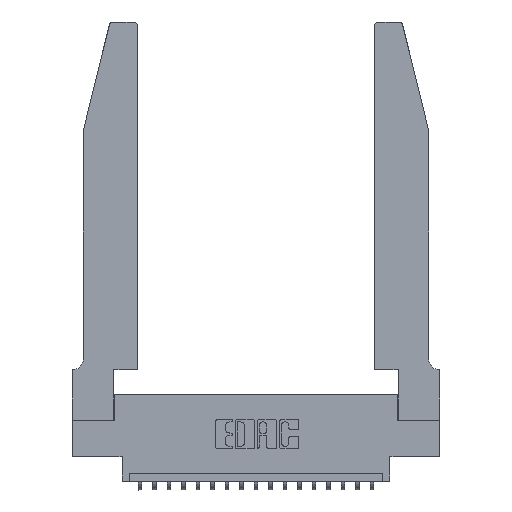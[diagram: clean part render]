
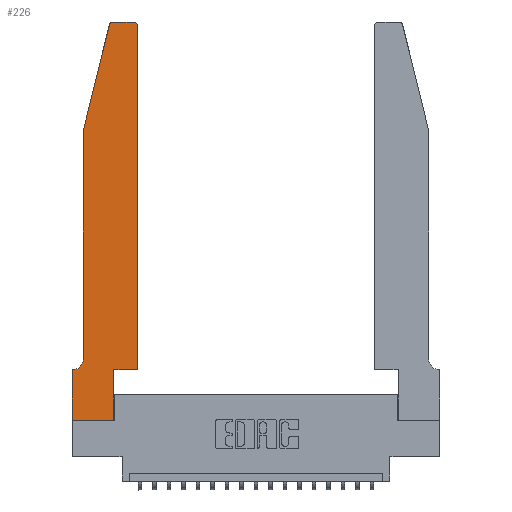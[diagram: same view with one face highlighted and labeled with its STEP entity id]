
A CAD part, top view. The second image highlights one B-rep face of the part: STEP entity #226.
In plain terms, the highlighted planar face has unit normal (0, 0, 1).
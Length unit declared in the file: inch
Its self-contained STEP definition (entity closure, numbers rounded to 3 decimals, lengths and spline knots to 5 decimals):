
#226 = ADVANCED_FACE ( 'NONE', ( #11697 ), #6208, .T. ) ;
#613 = CARTESIAN_POINT ( 'NONE',  ( 0.0055, 0.35, 0.37 ) ) ;
#615 = CARTESIAN_POINT ( 'NONE',  ( 0.4205, 2.75, 0.37 ) ) ;
#925 = DIRECTION ( 'NONE',  ( 0., 1., 0. ) ) ;
#1300 = CARTESIAN_POINT ( 'NONE',  ( 0.0755, 0.42, 0.37 ) ) ;
#1476 = AXIS2_PLACEMENT_3D ( 'NONE', #11097, #6129, #6274 ) ;
#2046 = ORIENTED_EDGE ( 'NONE', *, *, #7264, .T. ) ;
#2271 = EDGE_CURVE ( 'NONE', #5523, #13299, #11342, .T. ) ;
#2970 = CARTESIAN_POINT ( 'NONE',  ( 0.0755, 2., 0.37 ) ) ;
#3034 = EDGE_CURVE ( 'NONE', #18035, #12375, #16430, .T. ) ;
#3980 = DIRECTION ( 'NONE',  ( 1., 0., 0. ) ) ;
#4087 = ORIENTED_EDGE ( 'NONE', *, *, #3034, .T. ) ;
#4186 = ORIENTED_EDGE ( 'NONE', *, *, #5608, .T. ) ;
#4310 = DIRECTION ( 'NONE',  ( -0.239, -0.971, 0. ) ) ;
#4737 = AXIS2_PLACEMENT_3D ( 'NONE', #21066, #17824, #17966 ) ;
#4845 = LINE ( 'NONE', #20355, #16316 ) ;
#5082 = VERTEX_POINT ( 'NONE', #18088 ) ;
#5119 = CARTESIAN_POINT ( 'NONE',  ( 0.2865, 0.35, 0.37 ) ) ;
#5195 = VERTEX_POINT ( 'NONE', #615 ) ;
#5199 = CARTESIAN_POINT ( 'NONE',  ( 0.0755, 2., 0.37 ) ) ;
#5523 = VERTEX_POINT ( 'NONE', #9458 ) ;
#5608 = EDGE_CURVE ( 'NONE', #5195, #18035, #19732, .T. ) ;
#6129 = DIRECTION ( 'NONE',  ( 0., 0., 1. ) ) ;
#6154 = CARTESIAN_POINT ( 'NONE',  ( 0.2605, 2.75, 0.37 ) ) ;
#6208 = PLANE ( 'NONE',  #1476 ) ;
#6274 = DIRECTION ( 'NONE',  ( 1., 0., 0. ) ) ;
#6572 = VECTOR ( 'NONE', #16482, 39.37008 ) ;
#6970 = EDGE_LOOP ( 'NONE', ( #4186, #4087, #14527, #18084, #9827, #10660, #20049, #9057, #2046, #7508, #20483, #15471 ) ) ;
#7264 = EDGE_CURVE ( 'NONE', #17575, #14048, #10728, .T. ) ;
#7508 = ORIENTED_EDGE ( 'NONE', *, *, #9519, .T. ) ;
#7567 = CARTESIAN_POINT ( 'NONE',  ( 0.4505, 0.35, 0.37 ) ) ;
#7809 = VECTOR ( 'NONE', #17360, 39.37008 ) ;
#7847 = DIRECTION ( 'NONE',  ( -1., 0., 0. ) ) ;
#8094 = LINE ( 'NONE', #14356, #10865 ) ;
#8796 = VECTOR ( 'NONE', #13707, 39.37008 ) ;
#9057 = ORIENTED_EDGE ( 'NONE', *, *, #14700, .T. ) ;
#9154 = CIRCLE ( 'NONE', #20271, 0.03 ) ;
#9458 = CARTESIAN_POINT ( 'NONE',  ( 0., 0.35, 0.37 ) ) ;
#9519 = EDGE_CURVE ( 'NONE', #14048, #14787, #10866, .T. ) ;
#9658 = EDGE_CURVE ( 'NONE', #12375, #13492, #13658, .T. ) ;
#9763 = CARTESIAN_POINT ( 'NONE',  ( 0., 0., 0.37 ) ) ;
#9827 = ORIENTED_EDGE ( 'NONE', *, *, #15705, .T. ) ;
#10105 = EDGE_CURVE ( 'NONE', #13569, #5523, #15954, .T. ) ;
#10660 = ORIENTED_EDGE ( 'NONE', *, *, #10105, .T. ) ;
#10682 = CARTESIAN_POINT ( 'NONE',  ( 0.0055, 0.42, 0.37 ) ) ;
#10728 = LINE ( 'NONE', #17204, #14271 ) ;
#10865 = VECTOR ( 'NONE', #19170, 39.37008 ) ;
#10866 = LINE ( 'NONE', #15691, #6572 ) ;
#11097 = CARTESIAN_POINT ( 'NONE',  ( 0., 0.35, 0.37 ) ) ;
#11342 = LINE ( 'NONE', #16961, #8796 ) ;
#11594 = CARTESIAN_POINT ( 'NONE',  ( 0.0755, 2., 0.37 ) ) ;
#11697 = FACE_OUTER_BOUND ( 'NONE', #6970, .T. ) ;
#12375 = VERTEX_POINT ( 'NONE', #19940 ) ;
#12574 = DIRECTION ( 'NONE',  ( 0., 0., -1. ) ) ;
#13299 = VERTEX_POINT ( 'NONE', #9763 ) ;
#13339 = DIRECTION ( 'NONE',  ( 1., 0., 0. ) ) ;
#13492 = VERTEX_POINT ( 'NONE', #11594 ) ;
#13569 = VERTEX_POINT ( 'NONE', #613 ) ;
#13658 = LINE ( 'NONE', #2970, #17514 ) ;
#13707 = DIRECTION ( 'NONE',  ( 0., -1., 0. ) ) ;
#13722 = DIRECTION ( 'NONE',  ( -1., 0., 0. ) ) ;
#13801 = EDGE_CURVE ( 'NONE', #13492, #17981, #19396, .T. ) ;
#14048 = VERTEX_POINT ( 'NONE', #5119 ) ;
#14195 = CARTESIAN_POINT ( 'NONE',  ( 0.0755, 0.35, 0.37 ) ) ;
#14271 = VECTOR ( 'NONE', #925, 39.37008 ) ;
#14356 = CARTESIAN_POINT ( 'NONE',  ( 0.4505, 0.35, 0.37 ) ) ;
#14474 = EDGE_CURVE ( 'NONE', #5082, #5195, #9154, .T. ) ;
#14527 = ORIENTED_EDGE ( 'NONE', *, *, #9658, .T. ) ;
#14700 = EDGE_CURVE ( 'NONE', #13299, #17575, #4845, .T. ) ;
#14787 = VERTEX_POINT ( 'NONE', #7567 ) ;
#15044 = VECTOR ( 'NONE', #16607, 39.37008 ) ;
#15136 = CARTESIAN_POINT ( 'NONE',  ( 0.4205, 2.72, 0.37 ) ) ;
#15247 = CIRCLE ( 'NONE', #15749, 0.07 ) ;
#15373 = VECTOR ( 'NONE', #13722, 39.37008 ) ;
#15471 = ORIENTED_EDGE ( 'NONE', *, *, #14474, .T. ) ;
#15691 = CARTESIAN_POINT ( 'NONE',  ( 0.4505, 0.35, 0.37 ) ) ;
#15705 = EDGE_CURVE ( 'NONE', #17981, #13569, #15247, .T. ) ;
#15749 = AXIS2_PLACEMENT_3D ( 'NONE', #10682, #12574, #7847 ) ;
#15954 = LINE ( 'NONE', #14195, #7809 ) ;
#16191 = CARTESIAN_POINT ( 'NONE',  ( 0.2865, 0., 0.37 ) ) ;
#16316 = VECTOR ( 'NONE', #3980, 39.37008 ) ;
#16430 = CIRCLE ( 'NONE', #4737, 0.03 ) ;
#16482 = DIRECTION ( 'NONE',  ( 1., 0., 0. ) ) ;
#16561 = EDGE_CURVE ( 'NONE', #14787, #5082, #8094, .T. ) ;
#16607 = DIRECTION ( 'NONE',  ( 0., -1., 0. ) ) ;
#16644 = DIRECTION ( 'NONE',  ( 0., 0., 1. ) ) ;
#16961 = CARTESIAN_POINT ( 'NONE',  ( 0., 0., 0.37 ) ) ;
#17204 = CARTESIAN_POINT ( 'NONE',  ( 0.2865, 0.35, 0.37 ) ) ;
#17360 = DIRECTION ( 'NONE',  ( -1., 0., 0. ) ) ;
#17514 = VECTOR ( 'NONE', #4310, 39.37008 ) ;
#17575 = VERTEX_POINT ( 'NONE', #16191 ) ;
#17824 = DIRECTION ( 'NONE',  ( 0., 0., 1. ) ) ;
#17966 = DIRECTION ( 'NONE',  ( 1., 0., 0. ) ) ;
#17981 = VERTEX_POINT ( 'NONE', #1300 ) ;
#18035 = VERTEX_POINT ( 'NONE', #19145 ) ;
#18084 = ORIENTED_EDGE ( 'NONE', *, *, #13801, .T. ) ;
#18088 = CARTESIAN_POINT ( 'NONE',  ( 0.4505, 2.72, 0.37 ) ) ;
#19145 = CARTESIAN_POINT ( 'NONE',  ( 0.284, 2.75, 0.37 ) ) ;
#19170 = DIRECTION ( 'NONE',  ( 0., 1., 0. ) ) ;
#19396 = LINE ( 'NONE', #5199, #15044 ) ;
#19732 = LINE ( 'NONE', #6154, #15373 ) ;
#19940 = CARTESIAN_POINT ( 'NONE',  ( 0.25487, 2.72718, 0.37 ) ) ;
#20049 = ORIENTED_EDGE ( 'NONE', *, *, #2271, .T. ) ;
#20271 = AXIS2_PLACEMENT_3D ( 'NONE', #15136, #16644, #13339 ) ;
#20355 = CARTESIAN_POINT ( 'NONE',  ( 0., 0., 0.37 ) ) ;
#20483 = ORIENTED_EDGE ( 'NONE', *, *, #16561, .T. ) ;
#21066 = CARTESIAN_POINT ( 'NONE',  ( 0.284, 2.72, 0.37 ) ) ;
